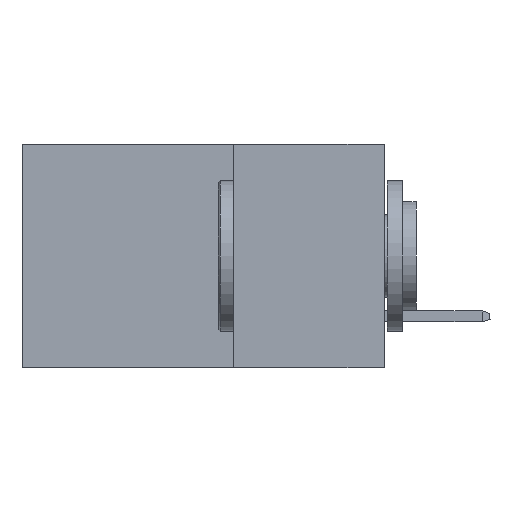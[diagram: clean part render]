
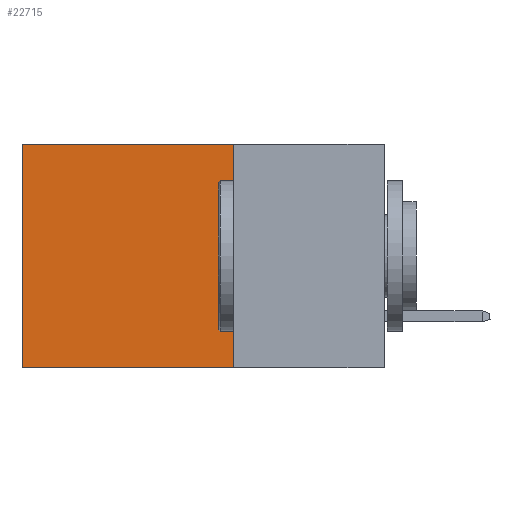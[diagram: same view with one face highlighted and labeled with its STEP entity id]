
A CAD part, left-side view. The second image highlights one B-rep face of the part: STEP entity #22715.
In plain terms, the highlighted planar face has unit normal (-1, 0, 0).
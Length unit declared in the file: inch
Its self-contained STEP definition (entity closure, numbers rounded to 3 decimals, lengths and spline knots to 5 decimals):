
#461 = LINE ( 'NONE', #19894, #7895 ) ;
#3003 = VECTOR ( 'NONE', #9351, 39.37008 ) ;
#5905 = CARTESIAN_POINT ( 'NONE',  ( 0.298, 0.25, 0. ) ) ;
#6044 = EDGE_CURVE ( 'NONE', #11647, #10354, #23703, .T. ) ;
#6445 = ORIENTED_EDGE ( 'NONE', *, *, #7585, .F. ) ;
#7197 = EDGE_CURVE ( 'NONE', #24541, #11647, #16478, .T. ) ;
#7585 = EDGE_CURVE ( 'NONE', #24541, #16821, #461, .T. ) ;
#7639 = EDGE_LOOP ( 'NONE', ( #23611, #16433, #6445, #15104 ) ) ;
#7687 = VECTOR ( 'NONE', #18842, 39.37008 ) ;
#7895 = VECTOR ( 'NONE', #22091, 39.37008 ) ;
#8238 = CARTESIAN_POINT ( 'NONE',  ( 0.298, 0.25, 0. ) ) ;
#9351 = DIRECTION ( 'NONE',  ( 0., 1., 0. ) ) ;
#9654 = CARTESIAN_POINT ( 'NONE',  ( 0.298, 0.6, -0.37 ) ) ;
#9815 = DIRECTION ( 'NONE',  ( 1., 0., 0. ) ) ;
#10126 = LINE ( 'NONE', #17807, #3003 ) ;
#10354 = VERTEX_POINT ( 'NONE', #9654 ) ;
#11647 = VERTEX_POINT ( 'NONE', #26860 ) ;
#12132 = EDGE_CURVE ( 'NONE', #16821, #10354, #10126, .T. ) ;
#12272 = AXIS2_PLACEMENT_3D ( 'NONE', #26316, #9815, #15927 ) ;
#15104 = ORIENTED_EDGE ( 'NONE', *, *, #7197, .T. ) ;
#15927 = DIRECTION ( 'NONE',  ( 0., 0., -1. ) ) ;
#16402 = DIRECTION ( 'NONE',  ( 0., 1., 0. ) ) ;
#16433 = ORIENTED_EDGE ( 'NONE', *, *, #12132, .F. ) ;
#16478 = LINE ( 'NONE', #8238, #26942 ) ;
#16821 = VERTEX_POINT ( 'NONE', #25220 ) ;
#17807 = CARTESIAN_POINT ( 'NONE',  ( 0.298, 0.25, -0.37 ) ) ;
#18582 = CARTESIAN_POINT ( 'NONE',  ( 0.298, 0.6, 0. ) ) ;
#18842 = DIRECTION ( 'NONE',  ( 0., 0., -1. ) ) ;
#19894 = CARTESIAN_POINT ( 'NONE',  ( 0.298, 0.25, 0. ) ) ;
#21996 = PLANE ( 'NONE',  #12272 ) ;
#22091 = DIRECTION ( 'NONE',  ( 0., 0., -1. ) ) ;
#22715 = ADVANCED_FACE ( 'NONE', ( #25452 ), #21996, .F. ) ;
#23611 = ORIENTED_EDGE ( 'NONE', *, *, #6044, .T. ) ;
#23703 = LINE ( 'NONE', #18582, #7687 ) ;
#24541 = VERTEX_POINT ( 'NONE', #5905 ) ;
#25220 = CARTESIAN_POINT ( 'NONE',  ( 0.298, 0.25, -0.37 ) ) ;
#25452 = FACE_OUTER_BOUND ( 'NONE', #7639, .T. ) ;
#26316 = CARTESIAN_POINT ( 'NONE',  ( 0.298, 0.25, 0. ) ) ;
#26860 = CARTESIAN_POINT ( 'NONE',  ( 0.298, 0.6, 0. ) ) ;
#26942 = VECTOR ( 'NONE', #16402, 39.37008 ) ;
